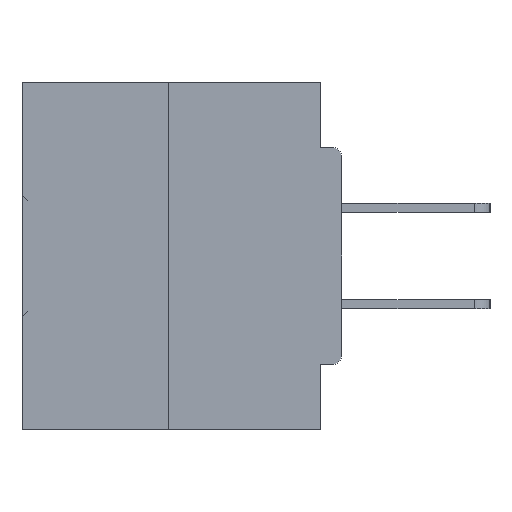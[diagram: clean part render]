
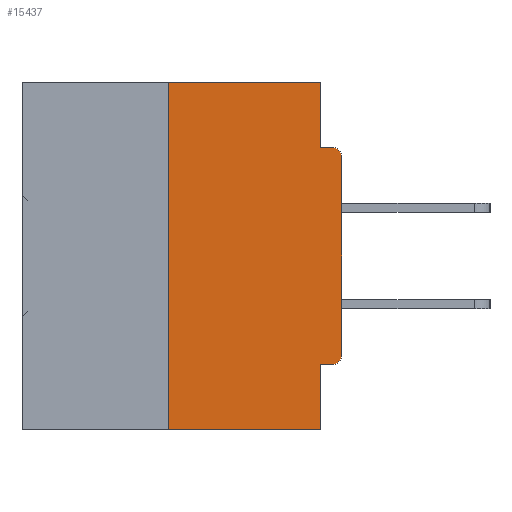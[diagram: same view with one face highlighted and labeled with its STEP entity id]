
A CAD part, left-side view. The second image highlights one B-rep face of the part: STEP entity #15437.
In plain terms, the highlighted planar face has unit normal (-1, 0, 0).
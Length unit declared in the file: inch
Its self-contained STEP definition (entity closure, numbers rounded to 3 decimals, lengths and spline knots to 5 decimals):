
#57 = VERTEX_POINT ( 'NONE', #3311 ) ;
#280 = EDGE_CURVE ( 'NONE', #46324, #30229, #45674, .T. ) ;
#702 = EDGE_CURVE ( 'NONE', #17605, #57, #22003, .T. ) ;
#926 = DIRECTION ( 'NONE',  ( 0., 0., -1. ) ) ;
#1323 = CARTESIAN_POINT ( 'NONE',  ( 0., 0.25, -0.5 ) ) ;
#2137 = CARTESIAN_POINT ( 'NONE',  ( 0., 0., -0.3915 ) ) ;
#2187 = EDGE_CURVE ( 'NONE', #34265, #46324, #23255, .T. ) ;
#2373 = ORIENTED_EDGE ( 'NONE', *, *, #280, .F. ) ;
#3311 = CARTESIAN_POINT ( 'NONE',  ( 0., 0.015, -0.0935 ) ) ;
#3506 = CARTESIAN_POINT ( 'NONE',  ( 0., 0.031, -0.5 ) ) ;
#5027 = CARTESIAN_POINT ( 'NONE',  ( 0., 0.25, 0. ) ) ;
#5896 = AXIS2_PLACEMENT_3D ( 'NONE', #33580, #29347, #926 ) ;
#5906 = CARTESIAN_POINT ( 'NONE',  ( 0., 0.031, -0.0935 ) ) ;
#6038 = VECTOR ( 'NONE', #45402, 39.37008 ) ;
#6642 = DIRECTION ( 'NONE',  ( 1., 0., 0. ) ) ;
#6726 = ORIENTED_EDGE ( 'NONE', *, *, #30128, .F. ) ;
#6989 = LINE ( 'NONE', #35640, #21614 ) ;
#7404 = DIRECTION ( 'NONE',  ( 0., -1., 0. ) ) ;
#7465 = ORIENTED_EDGE ( 'NONE', *, *, #23210, .T. ) ;
#7743 = CARTESIAN_POINT ( 'NONE',  ( 0., 0., -0.4065 ) ) ;
#8022 = CARTESIAN_POINT ( 'NONE',  ( 0., 0.25, 0. ) ) ;
#9459 = DIRECTION ( 'NONE',  ( 0., -1., 0. ) ) ;
#9679 = CIRCLE ( 'NONE', #5896, 0.015 ) ;
#11503 = ORIENTED_EDGE ( 'NONE', *, *, #702, .T. ) ;
#13662 = CARTESIAN_POINT ( 'NONE',  ( 0., 0.015, -0.1085 ) ) ;
#14841 = VERTEX_POINT ( 'NONE', #29751 ) ;
#15437 = ADVANCED_FACE ( 'NONE', ( #42399 ), #35281, .F. ) ;
#17605 = VERTEX_POINT ( 'NONE', #35318 ) ;
#17643 = DIRECTION ( 'NONE',  ( 0., 0., 1. ) ) ;
#19482 = DIRECTION ( 'NONE',  ( 0., 0., 1. ) ) ;
#19995 = EDGE_CURVE ( 'NONE', #14841, #43352, #9679, .T. ) ;
#20812 = VECTOR ( 'NONE', #28470, 39.37008 ) ;
#21299 = CARTESIAN_POINT ( 'NONE',  ( 0., 0.46, 0. ) ) ;
#21614 = VECTOR ( 'NONE', #17643, 39.37008 ) ;
#22003 = CIRCLE ( 'NONE', #37893, 0.015 ) ;
#22677 = CARTESIAN_POINT ( 'NONE',  ( 0., 0.031, -0.4065 ) ) ;
#23210 = EDGE_CURVE ( 'NONE', #34265, #28444, #42682, .T. ) ;
#23255 = LINE ( 'NONE', #5027, #36296 ) ;
#23570 = ORIENTED_EDGE ( 'NONE', *, *, #19995, .T. ) ;
#23602 = LINE ( 'NONE', #30970, #6038 ) ;
#24856 = DIRECTION ( 'NONE',  ( 0., 0., -1. ) ) ;
#25025 = LINE ( 'NONE', #7743, #26813 ) ;
#25390 = CARTESIAN_POINT ( 'NONE',  ( 0., 0., -0.0935 ) ) ;
#26813 = VECTOR ( 'NONE', #32844, 39.37008 ) ;
#26842 = CARTESIAN_POINT ( 'NONE',  ( 0., 0.031, -0.5 ) ) ;
#27510 = ORIENTED_EDGE ( 'NONE', *, *, #34053, .F. ) ;
#27602 = ORIENTED_EDGE ( 'NONE', *, *, #31486, .T. ) ;
#27632 = ORIENTED_EDGE ( 'NONE', *, *, #39976, .F. ) ;
#28302 = ORIENTED_EDGE ( 'NONE', *, *, #2187, .F. ) ;
#28444 = VERTEX_POINT ( 'NONE', #26842 ) ;
#28470 = DIRECTION ( 'NONE',  ( 0., -1., 0. ) ) ;
#29347 = DIRECTION ( 'NONE',  ( -1., 0., 0. ) ) ;
#29480 = VERTEX_POINT ( 'NONE', #5906 ) ;
#29751 = CARTESIAN_POINT ( 'NONE',  ( 0., 0.015, -0.4065 ) ) ;
#30128 = EDGE_CURVE ( 'NONE', #29480, #57, #39835, .T. ) ;
#30229 = VERTEX_POINT ( 'NONE', #45021 ) ;
#30970 = CARTESIAN_POINT ( 'NONE',  ( 0., 0.031, 0. ) ) ;
#31486 = EDGE_CURVE ( 'NONE', #43352, #17605, #6989, .T. ) ;
#31709 = LINE ( 'NONE', #3506, #46630 ) ;
#32609 = EDGE_CURVE ( 'NONE', #45089, #28444, #31709, .T. ) ;
#32844 = DIRECTION ( 'NONE',  ( 0., 1., 0. ) ) ;
#33580 = CARTESIAN_POINT ( 'NONE',  ( 0., 0.015, -0.3915 ) ) ;
#33758 = ORIENTED_EDGE ( 'NONE', *, *, #32609, .F. ) ;
#34053 = EDGE_CURVE ( 'NONE', #30229, #29480, #23602, .T. ) ;
#34190 = EDGE_LOOP ( 'NONE', ( #2373, #28302, #7465, #33758, #27632, #23570, #27602, #11503, #6726, #27510 ) ) ;
#34265 = VERTEX_POINT ( 'NONE', #1323 ) ;
#34732 = DIRECTION ( 'NONE',  ( 0., 0., -1. ) ) ;
#35281 = PLANE ( 'NONE',  #41849 ) ;
#35318 = CARTESIAN_POINT ( 'NONE',  ( 0., 0., -0.1085 ) ) ;
#35640 = CARTESIAN_POINT ( 'NONE',  ( 0., 0., 0. ) ) ;
#36296 = VECTOR ( 'NONE', #19482, 39.37008 ) ;
#37043 = VECTOR ( 'NONE', #9459, 39.37008 ) ;
#37370 = VECTOR ( 'NONE', #7404, 39.37008 ) ;
#37893 = AXIS2_PLACEMENT_3D ( 'NONE', #13662, #45391, #34732 ) ;
#39728 = DIRECTION ( 'NONE',  ( 0., 0., -1. ) ) ;
#39835 = LINE ( 'NONE', #25390, #37370 ) ;
#39976 = EDGE_CURVE ( 'NONE', #14841, #45089, #25025, .T. ) ;
#41849 = AXIS2_PLACEMENT_3D ( 'NONE', #21299, #6642, #24856 ) ;
#42355 = CARTESIAN_POINT ( 'NONE',  ( 0., 0.46, 0. ) ) ;
#42399 = FACE_OUTER_BOUND ( 'NONE', #34190, .T. ) ;
#42682 = LINE ( 'NONE', #46006, #20812 ) ;
#43352 = VERTEX_POINT ( 'NONE', #2137 ) ;
#45021 = CARTESIAN_POINT ( 'NONE',  ( 0., 0.031, 0. ) ) ;
#45089 = VERTEX_POINT ( 'NONE', #22677 ) ;
#45391 = DIRECTION ( 'NONE',  ( -1., 0., 0. ) ) ;
#45402 = DIRECTION ( 'NONE',  ( 0., 0., -1. ) ) ;
#45674 = LINE ( 'NONE', #42355, #37043 ) ;
#46006 = CARTESIAN_POINT ( 'NONE',  ( 0., 0.46, -0.5 ) ) ;
#46324 = VERTEX_POINT ( 'NONE', #8022 ) ;
#46630 = VECTOR ( 'NONE', #39728, 39.37008 ) ;
